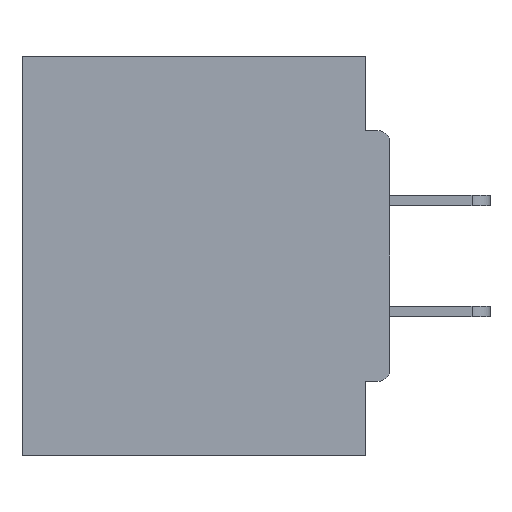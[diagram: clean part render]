
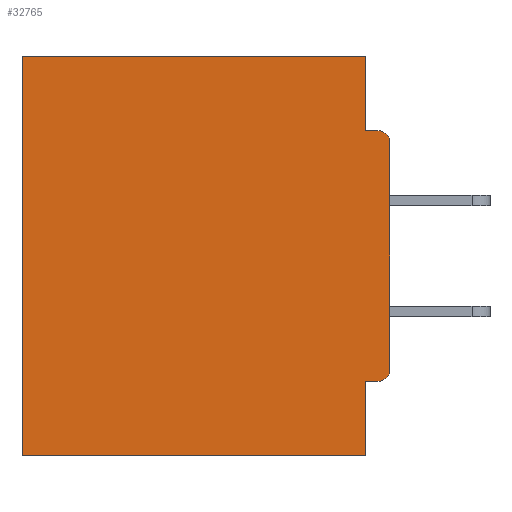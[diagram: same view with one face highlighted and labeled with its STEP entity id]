
A CAD part, left-side view. The second image highlights one B-rep face of the part: STEP entity #32765.
In plain terms, the highlighted planar face has unit normal (-1, 0, 0).
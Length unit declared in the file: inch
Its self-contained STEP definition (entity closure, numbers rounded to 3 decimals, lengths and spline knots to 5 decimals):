
#39 = EDGE_CURVE ( 'NONE', #8820, #3137, #13178, .T. ) ;
#285 = VERTEX_POINT ( 'NONE', #29524 ) ;
#1533 = ORIENTED_EDGE ( 'NONE', *, *, #14016, .F. ) ;
#1694 = DIRECTION ( 'NONE',  ( 0., 1., 0. ) ) ;
#3085 = VERTEX_POINT ( 'NONE', #12949 ) ;
#3137 = VERTEX_POINT ( 'NONE', #29617 ) ;
#3986 = CARTESIAN_POINT ( 'NONE',  ( 0.298, 0., 0. ) ) ;
#4645 = ORIENTED_EDGE ( 'NONE', *, *, #39, .T. ) ;
#4955 = ORIENTED_EDGE ( 'NONE', *, *, #25741, .F. ) ;
#5175 = ORIENTED_EDGE ( 'NONE', *, *, #7077, .T. ) ;
#5751 = ORIENTED_EDGE ( 'NONE', *, *, #22633, .F. ) ;
#6321 = EDGE_CURVE ( 'NONE', #3085, #20925, #29917, .T. ) ;
#6578 = EDGE_CURVE ( 'NONE', #20831, #25487, #13475, .T. ) ;
#6957 = VECTOR ( 'NONE', #1694, 39.37008 ) ;
#7077 = EDGE_CURVE ( 'NONE', #3137, #20676, #29700, .T. ) ;
#7613 = LINE ( 'NONE', #23937, #11358 ) ;
#8155 = DIRECTION ( 'NONE',  ( 0., 0., -1. ) ) ;
#8820 = VERTEX_POINT ( 'NONE', #32259 ) ;
#8826 = CARTESIAN_POINT ( 'NONE',  ( 0.298, 0., -0.4065 ) ) ;
#9339 = AXIS2_PLACEMENT_3D ( 'NONE', #3986, #25283, #14675 ) ;
#11093 = CARTESIAN_POINT ( 'NONE',  ( 0.298, 0.031, -0.5 ) ) ;
#11208 = CARTESIAN_POINT ( 'NONE',  ( 0.298, 0.031, -0.4065 ) ) ;
#11216 = DIRECTION ( 'NONE',  ( 0., 0., -1. ) ) ;
#11358 = VECTOR ( 'NONE', #23581, 39.37008 ) ;
#11731 = DIRECTION ( 'NONE',  ( 0., 0., -1. ) ) ;
#12564 = VERTEX_POINT ( 'NONE', #18080 ) ;
#12703 = AXIS2_PLACEMENT_3D ( 'NONE', #13404, #26469, #8155 ) ;
#12904 = LINE ( 'NONE', #19924, #32489 ) ;
#12949 = CARTESIAN_POINT ( 'NONE',  ( 0.298, 0., -0.1085 ) ) ;
#12973 = CARTESIAN_POINT ( 'NONE',  ( 0.298, 0., 0. ) ) ;
#13178 = LINE ( 'NONE', #33591, #6957 ) ;
#13404 = CARTESIAN_POINT ( 'NONE',  ( 0.298, 0.015, -0.3915 ) ) ;
#13475 = LINE ( 'NONE', #8826, #23069 ) ;
#13750 = EDGE_CURVE ( 'NONE', #8820, #12564, #12904, .T. ) ;
#14016 = EDGE_CURVE ( 'NONE', #3085, #30976, #24559, .T. ) ;
#14134 = VECTOR ( 'NONE', #26385, 39.37008 ) ;
#14675 = DIRECTION ( 'NONE',  ( 0., 0., -1. ) ) ;
#16201 = ORIENTED_EDGE ( 'NONE', *, *, #13750, .F. ) ;
#16948 = VECTOR ( 'NONE', #11216, 39.37008 ) ;
#17286 = FACE_OUTER_BOUND ( 'NONE', #30071, .T. ) ;
#17347 = CARTESIAN_POINT ( 'NONE',  ( 0.298, 0.46, -0.5 ) ) ;
#17586 = LINE ( 'NONE', #18658, #30910 ) ;
#18080 = CARTESIAN_POINT ( 'NONE',  ( 0.298, 0.031, -0.0935 ) ) ;
#18150 = DIRECTION ( 'NONE',  ( -1., 0., 0. ) ) ;
#18153 = CARTESIAN_POINT ( 'NONE',  ( 0.298, 0.015, -0.4065 ) ) ;
#18323 = ORIENTED_EDGE ( 'NONE', *, *, #6578, .F. ) ;
#18658 = CARTESIAN_POINT ( 'NONE',  ( 0.298, 0., -0.0935 ) ) ;
#18706 = ORIENTED_EDGE ( 'NONE', *, *, #20267, .T. ) ;
#19578 = DIRECTION ( 'NONE',  ( 0., 1., 0. ) ) ;
#19924 = CARTESIAN_POINT ( 'NONE',  ( 0.298, 0.031, -0.5 ) ) ;
#20267 = EDGE_CURVE ( 'NONE', #20831, #30976, #23387, .T. ) ;
#20629 = CARTESIAN_POINT ( 'NONE',  ( 0.298, 0.015, -0.1085 ) ) ;
#20676 = VERTEX_POINT ( 'NONE', #17347 ) ;
#20831 = VERTEX_POINT ( 'NONE', #18153 ) ;
#20925 = VERTEX_POINT ( 'NONE', #23666 ) ;
#21971 = LINE ( 'NONE', #11093, #16948 ) ;
#21995 = ORIENTED_EDGE ( 'NONE', *, *, #25278, .F. ) ;
#22633 = EDGE_CURVE ( 'NONE', #25487, #285, #21971, .T. ) ;
#23069 = VECTOR ( 'NONE', #19578, 39.37008 ) ;
#23281 = DIRECTION ( 'NONE',  ( 0., 0., -1. ) ) ;
#23387 = CIRCLE ( 'NONE', #12703, 0.015 ) ;
#23581 = DIRECTION ( 'NONE',  ( 0., 1., 0. ) ) ;
#23666 = CARTESIAN_POINT ( 'NONE',  ( 0.298, 0.015, -0.0935 ) ) ;
#23937 = CARTESIAN_POINT ( 'NONE',  ( 0.298, 0., -0.5 ) ) ;
#24559 = LINE ( 'NONE', #12973, #14134 ) ;
#25278 = EDGE_CURVE ( 'NONE', #285, #20676, #7613, .T. ) ;
#25283 = DIRECTION ( 'NONE',  ( 1., 0., 0. ) ) ;
#25487 = VERTEX_POINT ( 'NONE', #11208 ) ;
#25556 = ORIENTED_EDGE ( 'NONE', *, *, #6321, .T. ) ;
#25741 = EDGE_CURVE ( 'NONE', #12564, #20925, #17586, .T. ) ;
#26033 = CARTESIAN_POINT ( 'NONE',  ( 0.298, 0., -0.3915 ) ) ;
#26231 = CARTESIAN_POINT ( 'NONE',  ( 0.298, 0.46, 0. ) ) ;
#26385 = DIRECTION ( 'NONE',  ( 0., 0., -1. ) ) ;
#26469 = DIRECTION ( 'NONE',  ( -1., 0., 0. ) ) ;
#27626 = PLANE ( 'NONE',  #9339 ) ;
#29370 = DIRECTION ( 'NONE',  ( 0., -1., 0. ) ) ;
#29524 = CARTESIAN_POINT ( 'NONE',  ( 0.298, 0.031, -0.5 ) ) ;
#29617 = CARTESIAN_POINT ( 'NONE',  ( 0.298, 0.46, 0. ) ) ;
#29700 = LINE ( 'NONE', #26231, #32583 ) ;
#29917 = CIRCLE ( 'NONE', #34175, 0.015 ) ;
#30071 = EDGE_LOOP ( 'NONE', ( #25556, #4955, #16201, #4645, #5175, #21995, #5751, #18323, #18706, #1533 ) ) ;
#30910 = VECTOR ( 'NONE', #29370, 39.37008 ) ;
#30976 = VERTEX_POINT ( 'NONE', #26033 ) ;
#31245 = DIRECTION ( 'NONE',  ( 0., 0., -1. ) ) ;
#32259 = CARTESIAN_POINT ( 'NONE',  ( 0.298, 0.031, 0. ) ) ;
#32489 = VECTOR ( 'NONE', #11731, 39.37008 ) ;
#32583 = VECTOR ( 'NONE', #31245, 39.37008 ) ;
#32765 = ADVANCED_FACE ( 'NONE', ( #17286 ), #27626, .F. ) ;
#33591 = CARTESIAN_POINT ( 'NONE',  ( 0.298, 0., 0. ) ) ;
#34175 = AXIS2_PLACEMENT_3D ( 'NONE', #20629, #18150, #23281 ) ;
